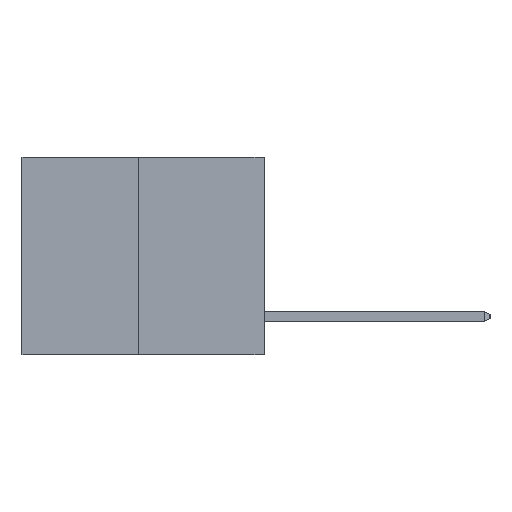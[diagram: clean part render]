
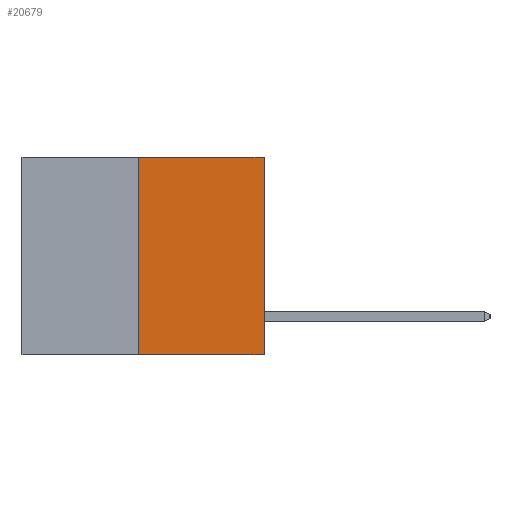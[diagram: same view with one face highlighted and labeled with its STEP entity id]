
A CAD part, left-side view. The second image highlights one B-rep face of the part: STEP entity #20679.
In plain terms, the highlighted planar face has unit normal (-1, 0, 0).
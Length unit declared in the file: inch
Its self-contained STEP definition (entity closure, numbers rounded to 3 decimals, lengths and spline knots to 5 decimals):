
#894 = ORIENTED_EDGE ( 'NONE', *, *, #11826, .T. ) ;
#1925 = AXIS2_PLACEMENT_3D ( 'NONE', #21329, #8043, #11338 ) ;
#3326 = VERTEX_POINT ( 'NONE', #10480 ) ;
#3924 = ORIENTED_EDGE ( 'NONE', *, *, #15965, .F. ) ;
#4498 = PLANE ( 'NONE',  #1925 ) ;
#4547 = DIRECTION ( 'NONE',  ( 0., -1., 0. ) ) ;
#5281 = VERTEX_POINT ( 'NONE', #12709 ) ;
#6353 = CARTESIAN_POINT ( 'NONE',  ( 0., 0.6, -0.49 ) ) ;
#6474 = EDGE_CURVE ( 'NONE', #8130, #5281, #15910, .T. ) ;
#6582 = ORIENTED_EDGE ( 'NONE', *, *, #6474, .F. ) ;
#6633 = CARTESIAN_POINT ( 'NONE',  ( 0., 0.312, -0.49 ) ) ;
#8043 = DIRECTION ( 'NONE',  ( 1., 0., 0. ) ) ;
#8095 = CARTESIAN_POINT ( 'NONE',  ( 0., 0.6, 0. ) ) ;
#8130 = VERTEX_POINT ( 'NONE', #15843 ) ;
#8950 = EDGE_CURVE ( 'NONE', #10735, #3326, #17571, .T. ) ;
#9818 = ORIENTED_EDGE ( 'NONE', *, *, #8950, .T. ) ;
#9876 = VECTOR ( 'NONE', #4547, 39.37008 ) ;
#10033 = VECTOR ( 'NONE', #17492, 39.37008 ) ;
#10480 = CARTESIAN_POINT ( 'NONE',  ( 0., 0., -0.49 ) ) ;
#10709 = LINE ( 'NONE', #14686, #19638 ) ;
#10735 = VERTEX_POINT ( 'NONE', #6633 ) ;
#11211 = DIRECTION ( 'NONE',  ( 0., -1., 0. ) ) ;
#11298 = VECTOR ( 'NONE', #11211, 39.37008 ) ;
#11338 = DIRECTION ( 'NONE',  ( 0., 0., -1. ) ) ;
#11826 = EDGE_CURVE ( 'NONE', #3326, #5281, #17891, .T. ) ;
#12709 = CARTESIAN_POINT ( 'NONE',  ( 0., 0., 0. ) ) ;
#14686 = CARTESIAN_POINT ( 'NONE',  ( 0., 0.312, -0.49 ) ) ;
#15843 = CARTESIAN_POINT ( 'NONE',  ( 0., 0.312, 0. ) ) ;
#15910 = LINE ( 'NONE', #8095, #9876 ) ;
#15965 = EDGE_CURVE ( 'NONE', #10735, #8130, #10709, .T. ) ;
#16111 = DIRECTION ( 'NONE',  ( 0., 0., 1. ) ) ;
#16335 = FACE_OUTER_BOUND ( 'NONE', #19559, .T. ) ;
#17492 = DIRECTION ( 'NONE',  ( 0., 0., 1. ) ) ;
#17571 = LINE ( 'NONE', #6353, #11298 ) ;
#17891 = LINE ( 'NONE', #20668, #10033 ) ;
#19559 = EDGE_LOOP ( 'NONE', ( #3924, #9818, #894, #6582 ) ) ;
#19638 = VECTOR ( 'NONE', #16111, 39.37008 ) ;
#20668 = CARTESIAN_POINT ( 'NONE',  ( 0., 0., 0. ) ) ;
#20679 = ADVANCED_FACE ( 'NONE', ( #16335 ), #4498, .F. ) ;
#21329 = CARTESIAN_POINT ( 'NONE',  ( 0., 0.6, 0. ) ) ;
